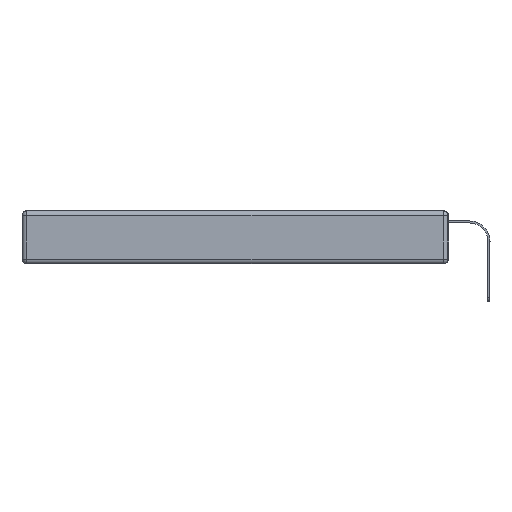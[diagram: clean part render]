
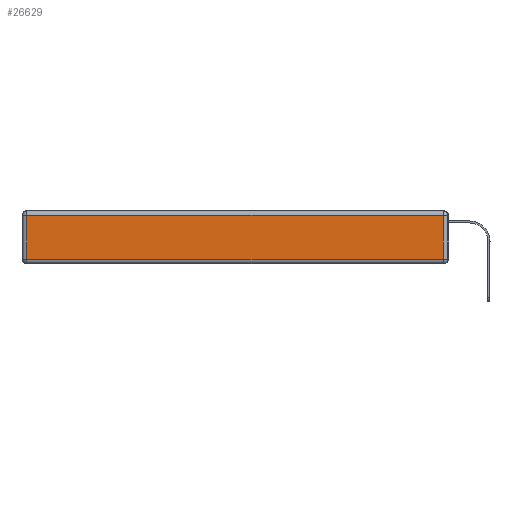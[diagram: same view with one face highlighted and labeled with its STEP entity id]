
A CAD part, left-side view. The second image highlights one B-rep face of the part: STEP entity #26629.
In plain terms, the highlighted planar face has unit normal (-1, 0, 0).
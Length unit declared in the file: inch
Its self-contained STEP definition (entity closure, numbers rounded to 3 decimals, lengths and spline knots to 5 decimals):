
#53 = ORIENTED_EDGE ( 'NONE', *, *, #18396, .T. ) ;
#2655 = LINE ( 'NONE', #11032, #5588 ) ;
#4251 = VECTOR ( 'NONE', #12659, 39.37008 ) ;
#4259 = VERTEX_POINT ( 'NONE', #9139 ) ;
#4460 = EDGE_LOOP ( 'NONE', ( #24351, #11465, #53, #19635 ) ) ;
#5588 = VECTOR ( 'NONE', #19417, 39.37008 ) ;
#5604 = VERTEX_POINT ( 'NONE', #26975 ) ;
#6638 = EDGE_CURVE ( 'NONE', #4259, #5604, #19326, .T. ) ;
#6824 = DIRECTION ( 'NONE',  ( 0., -1., 0. ) ) ;
#7632 = CARTESIAN_POINT ( 'NONE',  ( 0., 0.03, -0.03 ) ) ;
#9051 = CARTESIAN_POINT ( 'NONE',  ( 0., 0., -0.343 ) ) ;
#9139 = CARTESIAN_POINT ( 'NONE',  ( 0., 2.72, -0.313 ) ) ;
#9720 = DIRECTION ( 'NONE',  ( 0., 1., 0. ) ) ;
#9750 = VERTEX_POINT ( 'NONE', #17792 ) ;
#10036 = EDGE_CURVE ( 'NONE', #5604, #23119, #10878, .T. ) ;
#10878 = LINE ( 'NONE', #14619, #4251 ) ;
#11032 = CARTESIAN_POINT ( 'NONE',  ( 0., 2.72, -0.343 ) ) ;
#11465 = ORIENTED_EDGE ( 'NONE', *, *, #10036, .T. ) ;
#12452 = LINE ( 'NONE', #13982, #16215 ) ;
#12659 = DIRECTION ( 'NONE',  ( 0., 0., 1. ) ) ;
#13456 = VECTOR ( 'NONE', #6824, 39.37008 ) ;
#13982 = CARTESIAN_POINT ( 'NONE',  ( 0., 2.75, -0.03 ) ) ;
#14349 = EDGE_CURVE ( 'NONE', #9750, #4259, #2655, .T. ) ;
#14619 = CARTESIAN_POINT ( 'NONE',  ( 0., 0.03, -0.343 ) ) ;
#15112 = FACE_OUTER_BOUND ( 'NONE', #4460, .T. ) ;
#15497 = CARTESIAN_POINT ( 'NONE',  ( 0., 0., -0.313 ) ) ;
#16215 = VECTOR ( 'NONE', #9720, 39.37008 ) ;
#17580 = DIRECTION ( 'NONE',  ( 0., 0., 1. ) ) ;
#17792 = CARTESIAN_POINT ( 'NONE',  ( 0., 2.72, -0.03 ) ) ;
#18396 = EDGE_CURVE ( 'NONE', #23119, #9750, #12452, .T. ) ;
#19326 = LINE ( 'NONE', #15497, #13456 ) ;
#19417 = DIRECTION ( 'NONE',  ( 0., 0., -1. ) ) ;
#19635 = ORIENTED_EDGE ( 'NONE', *, *, #14349, .T. ) ;
#20729 = AXIS2_PLACEMENT_3D ( 'NONE', #9051, #21964, #17580 ) ;
#21830 = PLANE ( 'NONE',  #20729 ) ;
#21964 = DIRECTION ( 'NONE',  ( -1., 0., 0. ) ) ;
#23119 = VERTEX_POINT ( 'NONE', #7632 ) ;
#24351 = ORIENTED_EDGE ( 'NONE', *, *, #6638, .T. ) ;
#26629 = ADVANCED_FACE ( 'NONE', ( #15112 ), #21830, .T. ) ;
#26975 = CARTESIAN_POINT ( 'NONE',  ( 0., 0.03, -0.313 ) ) ;
